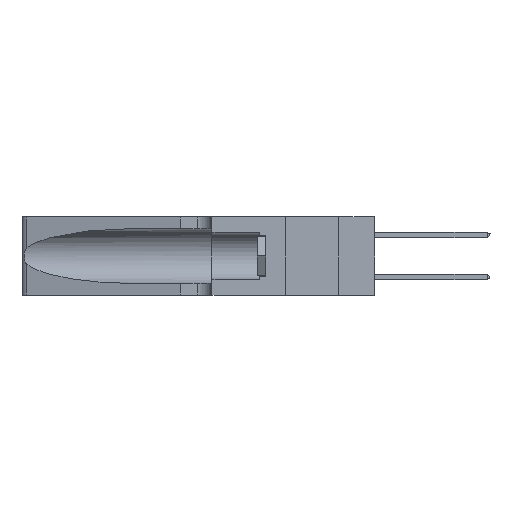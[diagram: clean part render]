
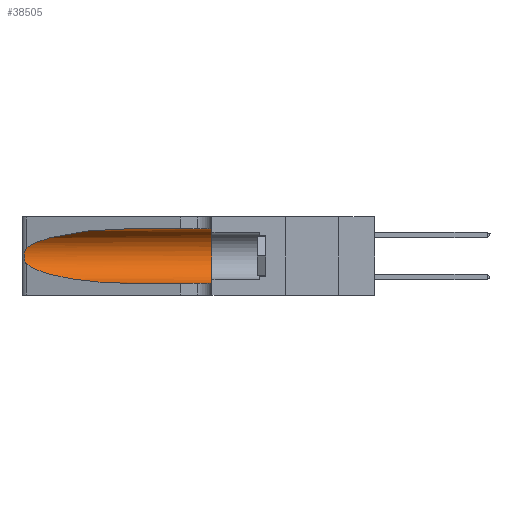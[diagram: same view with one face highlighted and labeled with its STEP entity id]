
A CAD part, left-side view. The second image highlights one B-rep face of the part: STEP entity #38505.
In plain terms, the highlighted cylindrical face has radius 3.308 mm (diameter 6.617 mm), a partial arc.
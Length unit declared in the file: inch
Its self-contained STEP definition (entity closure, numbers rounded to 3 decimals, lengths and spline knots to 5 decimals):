
#119 = CARTESIAN_POINT ( 'NONE',  ( 0.1305, 0.72297, 0.31525 ) ) ;
#515 = AXIS2_PLACEMENT_3D ( 'NONE', #5546, #8591, #27356 ) ;
#1088 = CARTESIAN_POINT ( 'NONE',  ( 0.25487, 1.22718, 0.22369 ) ) ;
#1111 = DIRECTION ( 'NONE',  ( 0., -1., 0. ) ) ;
#1154 = VECTOR ( 'NONE', #23404, 39.37008 ) ;
#1333 = CARTESIAN_POINT ( 'NONE',  ( 0.25487, 1.22718, 0.22369 ) ) ;
#1480 = CARTESIAN_POINT ( 'NONE',  ( 0.25555, 1.22993, 0.14849 ) ) ;
#1666 = CARTESIAN_POINT ( 'NONE',  ( 0.1305, 0.72297, 0.05475 ) ) ;
#2465 = EDGE_CURVE ( 'NONE', #28070, #12729, #38960, .T. ) ;
#4468 = FACE_OUTER_BOUND ( 'NONE', #19578, .T. ) ;
#4568 = CARTESIAN_POINT ( 'NONE',  ( 0.25555, 1.22994, 0.2215 ) ) ;
#5546 = CARTESIAN_POINT ( 'NONE',  ( 0.1305, 1.61858, 0.185 ) ) ;
#6164 = CARTESIAN_POINT ( 'NONE',  ( 0.25487, 1.22718, 0.22369 ) ) ;
#6205 = VERTEX_POINT ( 'NONE', #1088 ) ;
#7483 = B_SPLINE_CURVE_WITH_KNOTS ( 'NONE', 3,
 ( #1333, #4568, #26383, #7722, #29489, #10922, #32620, #14033, #35774, #17158, #38910, #20281, #1480, #23412 ),
 .UNSPECIFIED., .F., .F.,
 ( 4, 2, 2, 2, 2, 2, 4 ),
 ( 0., 0.00027, 0.00053, 0.00107, 0.0016, 0.00187, 0.00214 ),
 .UNSPECIFIED. ) ;
#7638 = DIRECTION ( 'NONE',  ( 0., 1., 0. ) ) ;
#7722 = CARTESIAN_POINT ( 'NONE',  ( 0.25787, 1.23484, 0.2124 ) ) ;
#7909 = CARTESIAN_POINT ( 'NONE',  ( 0.25487, 1.22718, 0.14631 ) ) ;
#8591 = DIRECTION ( 'NONE',  ( 0., -1., 0. ) ) ;
#9508 = LINE ( 'NONE', #16664, #22178 ) ;
#9940 = ORIENTED_EDGE ( 'NONE', *, *, #2465, .F. ) ;
#10922 = CARTESIAN_POINT ( 'NONE',  ( 0.26018, 1.23835, 0.19895 ) ) ;
#12729 = VERTEX_POINT ( 'NONE', #38565 ) ;
#14033 = CARTESIAN_POINT ( 'NONE',  ( 0.26075, 1.23896, 0.178 ) ) ;
#14759 =( BOUNDED_CURVE ( )  B_SPLINE_CURVE ( 3, ( #7909, #32805, #20459, #1666 ),
 .UNSPECIFIED., .F., .T. ) 
 B_SPLINE_CURVE_WITH_KNOTS ( ( 4, 4 ),
 ( 3.44316, 4.71239 ),
 .UNSPECIFIED. ) 
 CURVE ( )  GEOMETRIC_REPRESENTATION_ITEM ( )  RATIONAL_B_SPLINE_CURVE ( ( 1., 0.87, 0.87, 1. ) ) 
 REPRESENTATION_ITEM ( '' )  );
#16664 = CARTESIAN_POINT ( 'NONE',  ( 0.1305, 1.61858, 0.31525 ) ) ;
#17158 = CARTESIAN_POINT ( 'NONE',  ( 0.25856, 1.23593, 0.16098 ) ) ;
#17604 = AXIS2_PLACEMENT_3D ( 'NONE', #26304, #7638, #29401 ) ;
#17893 = LINE ( 'NONE', #20272, #1154 ) ;
#18605 = CARTESIAN_POINT ( 'NONE',  ( 0.1305, 0.72297, 0.31525 ) ) ;
#19578 = EDGE_LOOP ( 'NONE', ( #27967, #39128, #40103, #33766, #9940, #20164 ) ) ;
#20164 = ORIENTED_EDGE ( 'NONE', *, *, #37576, .F. ) ;
#20272 = CARTESIAN_POINT ( 'NONE',  ( 0.1305, 1.61858, 0.05475 ) ) ;
#20281 = CARTESIAN_POINT ( 'NONE',  ( 0.25639, 1.23186, 0.15144 ) ) ;
#20459 = CARTESIAN_POINT ( 'NONE',  ( 0.18966, 0.96281, 0.05475 ) ) ;
#22017 =( BOUNDED_CURVE ( )  B_SPLINE_CURVE ( 3, ( #18605, #37226, #24850, #6164 ),
 .UNSPECIFIED., .F., .T. ) 
 B_SPLINE_CURVE_WITH_KNOTS ( ( 4, 4 ),
 ( 1.5708, 2.84003 ),
 .UNSPECIFIED. ) 
 CURVE ( )  GEOMETRIC_REPRESENTATION_ITEM ( )  RATIONAL_B_SPLINE_CURVE ( ( 1., 0.87, 0.87, 1. ) ) 
 REPRESENTATION_ITEM ( '' )  );
#22178 = VECTOR ( 'NONE', #1111, 39.37008 ) ;
#23404 = DIRECTION ( 'NONE',  ( 0., -1., 0. ) ) ;
#23412 = CARTESIAN_POINT ( 'NONE',  ( 0.25487, 1.22718, 0.14631 ) ) ;
#23869 = VERTEX_POINT ( 'NONE', #119 ) ;
#24850 = CARTESIAN_POINT ( 'NONE',  ( 0.2373, 1.15595, 0.28018 ) ) ;
#26304 = CARTESIAN_POINT ( 'NONE',  ( 0.1305, 0.35, 0.185 ) ) ;
#26383 = CARTESIAN_POINT ( 'NONE',  ( 0.25639, 1.23184, 0.21858 ) ) ;
#27356 = DIRECTION ( 'NONE',  ( 0., 0., -1. ) ) ;
#27426 = VERTEX_POINT ( 'NONE', #35251 ) ;
#27967 = ORIENTED_EDGE ( 'NONE', *, *, #29915, .T. ) ;
#28070 = VERTEX_POINT ( 'NONE', #35071 ) ;
#28375 = CYLINDRICAL_SURFACE ( 'NONE', #515, 0.13025 ) ;
#29002 = EDGE_CURVE ( 'NONE', #37218, #12729, #17893, .T. ) ;
#29401 = DIRECTION ( 'NONE',  ( 0., 0., 1. ) ) ;
#29489 = CARTESIAN_POINT ( 'NONE',  ( 0.25854, 1.2359, 0.20912 ) ) ;
#29915 = EDGE_CURVE ( 'NONE', #23869, #6205, #22017, .T. ) ;
#30315 = EDGE_CURVE ( 'NONE', #27426, #37218, #14759, .T. ) ;
#30784 = CARTESIAN_POINT ( 'NONE',  ( 0.1305, 0.72297, 0.05475 ) ) ;
#30920 = EDGE_CURVE ( 'NONE', #6205, #27426, #7483, .T. ) ;
#32620 = CARTESIAN_POINT ( 'NONE',  ( 0.26075, 1.23896, 0.19203 ) ) ;
#32805 = CARTESIAN_POINT ( 'NONE',  ( 0.2373, 1.15595, 0.08982 ) ) ;
#33766 = ORIENTED_EDGE ( 'NONE', *, *, #29002, .T. ) ;
#35071 = CARTESIAN_POINT ( 'NONE',  ( 0.1305, 0.35, 0.31525 ) ) ;
#35251 = CARTESIAN_POINT ( 'NONE',  ( 0.25487, 1.22718, 0.14631 ) ) ;
#35774 = CARTESIAN_POINT ( 'NONE',  ( 0.26017, 1.23833, 0.17102 ) ) ;
#37218 = VERTEX_POINT ( 'NONE', #30784 ) ;
#37226 = CARTESIAN_POINT ( 'NONE',  ( 0.18966, 0.96281, 0.31525 ) ) ;
#37576 = EDGE_CURVE ( 'NONE', #23869, #28070, #9508, .T. ) ;
#38505 = ADVANCED_FACE ( 'NONE', ( #4468 ), #28375, .F. ) ;
#38565 = CARTESIAN_POINT ( 'NONE',  ( 0.1305, 0.35, 0.05475 ) ) ;
#38910 = CARTESIAN_POINT ( 'NONE',  ( 0.25789, 1.23486, 0.15765 ) ) ;
#38960 = CIRCLE ( 'NONE', #17604, 0.13025 ) ;
#39128 = ORIENTED_EDGE ( 'NONE', *, *, #30920, .T. ) ;
#40103 = ORIENTED_EDGE ( 'NONE', *, *, #30315, .T. ) ;
